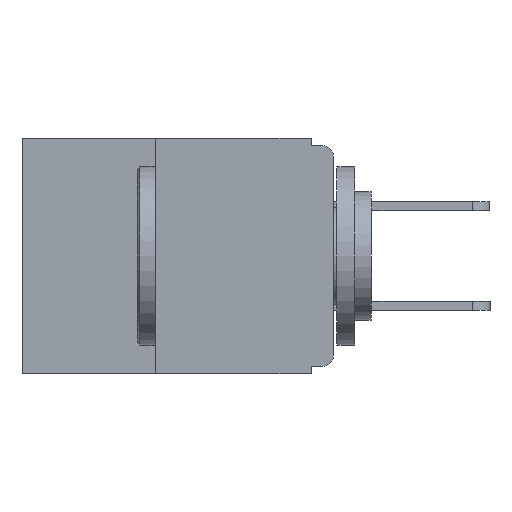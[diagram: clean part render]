
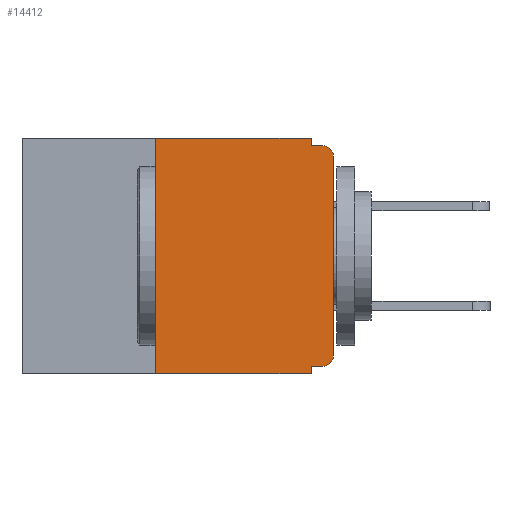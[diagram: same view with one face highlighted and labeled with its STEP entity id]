
A CAD part, left-side view. The second image highlights one B-rep face of the part: STEP entity #14412.
In plain terms, the highlighted planar face has unit normal (-1, 0, 0).
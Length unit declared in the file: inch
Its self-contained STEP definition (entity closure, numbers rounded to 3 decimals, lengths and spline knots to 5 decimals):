
#26 = DIRECTION ( 'NONE',  ( 0., 1., 0. ) ) ;
#42 = DIRECTION ( 'NONE',  ( 0., 0., -1. ) ) ;
#183 = VERTEX_POINT ( 'NONE', #4007 ) ;
#214 = DIRECTION ( 'NONE',  ( -1., 0., 0. ) ) ;
#240 = CARTESIAN_POINT ( 'NONE',  ( 0., 0.031, -0.01 ) ) ;
#244 = CARTESIAN_POINT ( 'NONE',  ( 0., 0.015, -0.305 ) ) ;
#757 = DIRECTION ( 'NONE',  ( 0., -1., 0. ) ) ;
#812 = CARTESIAN_POINT ( 'NONE',  ( 0., 0.437, 0. ) ) ;
#889 = DIRECTION ( 'NONE',  ( 1., 0., 0. ) ) ;
#1190 = CARTESIAN_POINT ( 'NONE',  ( 0., 0.031, -0.32 ) ) ;
#1304 = EDGE_CURVE ( 'NONE', #17847, #15222, #17756, .T. ) ;
#1700 = LINE ( 'NONE', #2180, #7222 ) ;
#1854 = CARTESIAN_POINT ( 'NONE',  ( 0., 0.25, 0. ) ) ;
#2051 = CARTESIAN_POINT ( 'NONE',  ( 0., 0.25, -0.33 ) ) ;
#2180 = CARTESIAN_POINT ( 'NONE',  ( 0., 0.031, 0. ) ) ;
#2236 = LINE ( 'NONE', #2667, #9957 ) ;
#2277 = ORIENTED_EDGE ( 'NONE', *, *, #11608, .T. ) ;
#2486 = VECTOR ( 'NONE', #42, 39.37008 ) ;
#2510 = ORIENTED_EDGE ( 'NONE', *, *, #11214, .F. ) ;
#2561 = AXIS2_PLACEMENT_3D ( 'NONE', #244, #214, #18587 ) ;
#2609 = ORIENTED_EDGE ( 'NONE', *, *, #14333, .F. ) ;
#2652 = CARTESIAN_POINT ( 'NONE',  ( 0., 0.031, -0.33 ) ) ;
#2667 = CARTESIAN_POINT ( 'NONE',  ( 0., 0., 0. ) ) ;
#3173 = EDGE_CURVE ( 'NONE', #17976, #183, #13546, .T. ) ;
#3448 = VECTOR ( 'NONE', #757, 39.37008 ) ;
#4007 = CARTESIAN_POINT ( 'NONE',  ( 0., 0.031, 0. ) ) ;
#4287 = EDGE_CURVE ( 'NONE', #15920, #12060, #18542, .T. ) ;
#5389 = CARTESIAN_POINT ( 'NONE',  ( 0., 0., -0.01 ) ) ;
#5850 = VECTOR ( 'NONE', #19239, 39.37008 ) ;
#6037 = EDGE_LOOP ( 'NONE', ( #12080, #2277, #2510, #2609, #11801, #18726, #15302, #8717, #18287, #18303 ) ) ;
#6050 = VECTOR ( 'NONE', #8245, 39.37008 ) ;
#6220 = VECTOR ( 'NONE', #26, 39.37008 ) ;
#6434 = VECTOR ( 'NONE', #11659, 39.37008 ) ;
#6670 = DIRECTION ( 'NONE',  ( -1., 0., 0. ) ) ;
#6895 = VERTEX_POINT ( 'NONE', #14447 ) ;
#6962 = EDGE_CURVE ( 'NONE', #6895, #12060, #18456, .T. ) ;
#7056 = CIRCLE ( 'NONE', #11522, 0.015 ) ;
#7222 = VECTOR ( 'NONE', #18828, 39.37008 ) ;
#7609 = CARTESIAN_POINT ( 'NONE',  ( 0., 0.031, -0.33 ) ) ;
#8245 = DIRECTION ( 'NONE',  ( 0., 0., 1. ) ) ;
#8677 = VERTEX_POINT ( 'NONE', #18365 ) ;
#8717 = ORIENTED_EDGE ( 'NONE', *, *, #4287, .F. ) ;
#9351 = CARTESIAN_POINT ( 'NONE',  ( 0., 0.015, -0.32 ) ) ;
#9957 = VECTOR ( 'NONE', #11868, 39.37008 ) ;
#10214 = LINE ( 'NONE', #2051, #6050 ) ;
#11214 = EDGE_CURVE ( 'NONE', #14646, #16230, #18581, .T. ) ;
#11522 = AXIS2_PLACEMENT_3D ( 'NONE', #15776, #6670, #17282 ) ;
#11608 = EDGE_CURVE ( 'NONE', #8677, #16230, #7056, .T. ) ;
#11659 = DIRECTION ( 'NONE',  ( 0., -1., 0. ) ) ;
#11673 = DIRECTION ( 'NONE',  ( 0., 0., -1. ) ) ;
#11801 = ORIENTED_EDGE ( 'NONE', *, *, #3173, .F. ) ;
#11868 = DIRECTION ( 'NONE',  ( 0., 0., 1. ) ) ;
#11872 = EDGE_CURVE ( 'NONE', #15222, #8677, #2236, .T. ) ;
#12060 = VERTEX_POINT ( 'NONE', #7609 ) ;
#12080 = ORIENTED_EDGE ( 'NONE', *, *, #11872, .T. ) ;
#12730 = CARTESIAN_POINT ( 'NONE',  ( 0., 0.437, -0.33 ) ) ;
#13546 = LINE ( 'NONE', #14509, #5850 ) ;
#13897 = CARTESIAN_POINT ( 'NONE',  ( 0., 0., -0.32 ) ) ;
#14333 = EDGE_CURVE ( 'NONE', #183, #14646, #1700, .T. ) ;
#14412 = ADVANCED_FACE ( 'NONE', ( #16474 ), #14596, .F. ) ;
#14447 = CARTESIAN_POINT ( 'NONE',  ( 0., 0.25, -0.33 ) ) ;
#14509 = CARTESIAN_POINT ( 'NONE',  ( 0., 0.437, 0. ) ) ;
#14596 = PLANE ( 'NONE',  #16827 ) ;
#14646 = VERTEX_POINT ( 'NONE', #240 ) ;
#15222 = VERTEX_POINT ( 'NONE', #18295 ) ;
#15302 = ORIENTED_EDGE ( 'NONE', *, *, #6962, .T. ) ;
#15776 = CARTESIAN_POINT ( 'NONE',  ( 0., 0.015, -0.025 ) ) ;
#15920 = VERTEX_POINT ( 'NONE', #1190 ) ;
#16230 = VERTEX_POINT ( 'NONE', #18560 ) ;
#16474 = FACE_OUTER_BOUND ( 'NONE', #6037, .T. ) ;
#16827 = AXIS2_PLACEMENT_3D ( 'NONE', #812, #889, #11673 ) ;
#17282 = DIRECTION ( 'NONE',  ( 0., 0., -1. ) ) ;
#17756 = CIRCLE ( 'NONE', #2561, 0.015 ) ;
#17847 = VERTEX_POINT ( 'NONE', #9351 ) ;
#17976 = VERTEX_POINT ( 'NONE', #1854 ) ;
#18066 = EDGE_CURVE ( 'NONE', #6895, #17976, #10214, .T. ) ;
#18287 = ORIENTED_EDGE ( 'NONE', *, *, #19477, .F. ) ;
#18295 = CARTESIAN_POINT ( 'NONE',  ( 0., 0., -0.305 ) ) ;
#18303 = ORIENTED_EDGE ( 'NONE', *, *, #1304, .T. ) ;
#18365 = CARTESIAN_POINT ( 'NONE',  ( 0., 0., -0.025 ) ) ;
#18456 = LINE ( 'NONE', #12730, #6434 ) ;
#18542 = LINE ( 'NONE', #2652, #2486 ) ;
#18560 = CARTESIAN_POINT ( 'NONE',  ( 0., 0.015, -0.01 ) ) ;
#18581 = LINE ( 'NONE', #5389, #3448 ) ;
#18587 = DIRECTION ( 'NONE',  ( 0., 0., -1. ) ) ;
#18726 = ORIENTED_EDGE ( 'NONE', *, *, #18066, .F. ) ;
#18728 = LINE ( 'NONE', #13897, #6220 ) ;
#18828 = DIRECTION ( 'NONE',  ( 0., 0., -1. ) ) ;
#19239 = DIRECTION ( 'NONE',  ( 0., -1., 0. ) ) ;
#19477 = EDGE_CURVE ( 'NONE', #17847, #15920, #18728, .T. ) ;
